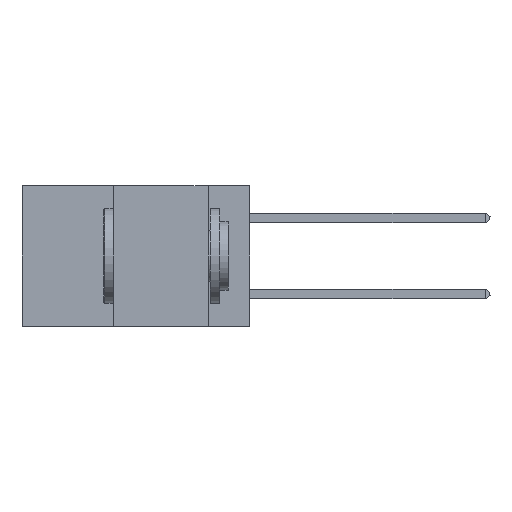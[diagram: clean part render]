
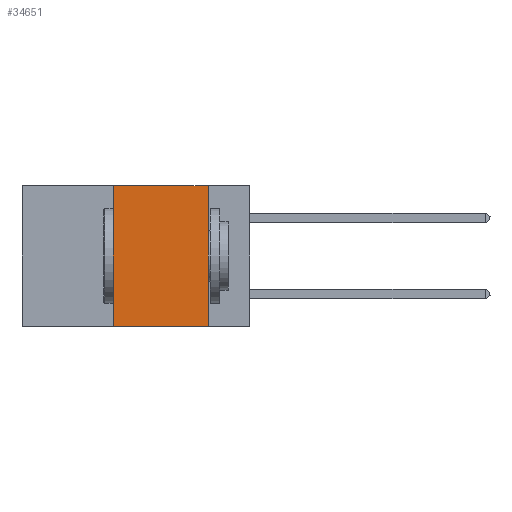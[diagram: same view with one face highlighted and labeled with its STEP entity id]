
A CAD part, left-side view. The second image highlights one B-rep face of the part: STEP entity #34651.
In plain terms, the highlighted planar face has unit normal (-1, 0, 0).
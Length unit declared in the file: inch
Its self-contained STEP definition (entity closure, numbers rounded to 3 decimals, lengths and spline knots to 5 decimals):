
#922 = PLANE ( 'NONE',  #3176 ) ;
#1467 = ORIENTED_EDGE ( 'NONE', *, *, #39927, .T. ) ;
#1578 = CARTESIAN_POINT ( 'NONE',  ( 0., 0.11, 0. ) ) ;
#3176 = AXIS2_PLACEMENT_3D ( 'NONE', #33570, #36822, #17313 ) ;
#4523 = VECTOR ( 'NONE', #7549, 39.37008 ) ;
#6472 = CARTESIAN_POINT ( 'NONE',  ( 0., 0.11, -0.37 ) ) ;
#7549 = DIRECTION ( 'NONE',  ( 0., 0., 1. ) ) ;
#7920 = CARTESIAN_POINT ( 'NONE',  ( 0., 0.11, 0. ) ) ;
#8180 = CARTESIAN_POINT ( 'NONE',  ( 0., 0.36, -0.37 ) ) ;
#8903 = LINE ( 'NONE', #14009, #20657 ) ;
#9920 = VECTOR ( 'NONE', #9949, 39.37008 ) ;
#9949 = DIRECTION ( 'NONE',  ( 0., -1., 0. ) ) ;
#10766 = ORIENTED_EDGE ( 'NONE', *, *, #20389, .F. ) ;
#10832 = VERTEX_POINT ( 'NONE', #15231 ) ;
#11494 = VERTEX_POINT ( 'NONE', #7920 ) ;
#13588 = EDGE_LOOP ( 'NONE', ( #26989, #10766, #20709, #1467 ) ) ;
#14009 = CARTESIAN_POINT ( 'NONE',  ( 0., 0.6, -0.37 ) ) ;
#14029 = LINE ( 'NONE', #40449, #9920 ) ;
#15231 = CARTESIAN_POINT ( 'NONE',  ( 0., 0.36, 0. ) ) ;
#15759 = VERTEX_POINT ( 'NONE', #6472 ) ;
#16198 = EDGE_CURVE ( 'NONE', #11494, #15759, #29097, .T. ) ;
#16743 = VECTOR ( 'NONE', #34511, 39.37008 ) ;
#17313 = DIRECTION ( 'NONE',  ( 0., 0., -1. ) ) ;
#17324 = EDGE_CURVE ( 'NONE', #25095, #10832, #21868, .T. ) ;
#20389 = EDGE_CURVE ( 'NONE', #10832, #11494, #14029, .T. ) ;
#20657 = VECTOR ( 'NONE', #39545, 39.37008 ) ;
#20709 = ORIENTED_EDGE ( 'NONE', *, *, #17324, .F. ) ;
#21868 = LINE ( 'NONE', #27148, #4523 ) ;
#25095 = VERTEX_POINT ( 'NONE', #8180 ) ;
#26989 = ORIENTED_EDGE ( 'NONE', *, *, #16198, .F. ) ;
#27148 = CARTESIAN_POINT ( 'NONE',  ( 0., 0.36, 0. ) ) ;
#29097 = LINE ( 'NONE', #1578, #16743 ) ;
#33570 = CARTESIAN_POINT ( 'NONE',  ( 0., 0.6, 0. ) ) ;
#34511 = DIRECTION ( 'NONE',  ( 0., 0., -1. ) ) ;
#34651 = ADVANCED_FACE ( 'NONE', ( #38640 ), #922, .F. ) ;
#36822 = DIRECTION ( 'NONE',  ( 1., 0., 0. ) ) ;
#38640 = FACE_OUTER_BOUND ( 'NONE', #13588, .T. ) ;
#39545 = DIRECTION ( 'NONE',  ( 0., -1., 0. ) ) ;
#39927 = EDGE_CURVE ( 'NONE', #25095, #15759, #8903, .T. ) ;
#40449 = CARTESIAN_POINT ( 'NONE',  ( 0., 0.6, 0. ) ) ;
